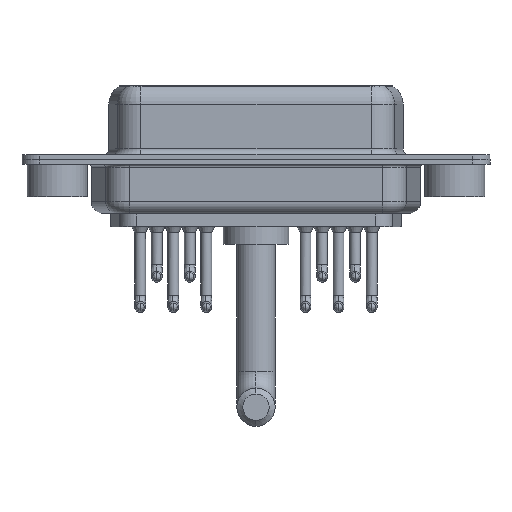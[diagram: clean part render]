
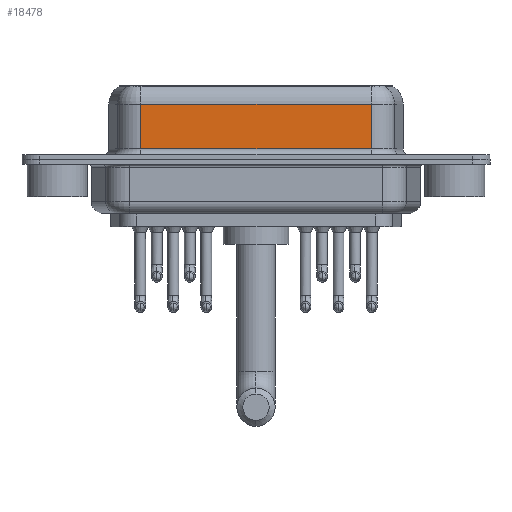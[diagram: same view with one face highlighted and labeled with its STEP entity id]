
A CAD part, front view. The second image highlights one B-rep face of the part: STEP entity #18478.
In plain terms, the highlighted planar face has unit normal (0, -1, 0).
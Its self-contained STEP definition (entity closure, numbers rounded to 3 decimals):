
#212 = VECTOR ( 'NONE', #18120, 1000. ) ;
#762 = CARTESIAN_POINT ( 'NONE',  ( 7.013, -3.95, 4.65 ) ) ;
#2503 = PLANE ( 'NONE',  #17498 ) ;
#2688 = VERTEX_POINT ( 'NONE', #15954 ) ;
#2879 = VERTEX_POINT ( 'NONE', #17060 ) ;
#2999 = EDGE_CURVE ( 'NONE', #7984, #10049, #8104, .T. ) ;
#3759 = ORIENTED_EDGE ( 'NONE', *, *, #16179, .F. ) ;
#4712 = CARTESIAN_POINT ( 'NONE',  ( 7.013, -3.95, 0.9 ) ) ;
#4787 = DIRECTION ( 'NONE',  ( -1., 0., 0. ) ) ;
#5198 = VECTOR ( 'NONE', #11987, 1000. ) ;
#5948 = EDGE_CURVE ( 'NONE', #2879, #7984, #13646, .T. ) ;
#6140 = LINE ( 'NONE', #17648, #5198 ) ;
#6589 = VECTOR ( 'NONE', #16693, 1000. ) ;
#6753 = FACE_OUTER_BOUND ( 'NONE', #17752, .T. ) ;
#7984 = VERTEX_POINT ( 'NONE', #762 ) ;
#8010 = LINE ( 'NONE', #13747, #6589 ) ;
#8104 = LINE ( 'NONE', #13842, #212 ) ;
#8258 = DIRECTION ( 'NONE',  ( 0., 1., 0. ) ) ;
#9667 = CARTESIAN_POINT ( 'NONE',  ( 26.287, -3.95, 6.4 ) ) ;
#10049 = VERTEX_POINT ( 'NONE', #4712 ) ;
#11621 = EDGE_CURVE ( 'NONE', #10049, #2688, #6140, .T. ) ;
#11987 = DIRECTION ( 'NONE',  ( 1., 0., 0. ) ) ;
#13646 = LINE ( 'NONE', #17723, #17110 ) ;
#13747 = CARTESIAN_POINT ( 'NONE',  ( 26.287, -3.95, 6.4 ) ) ;
#13842 = CARTESIAN_POINT ( 'NONE',  ( 7.013, -3.95, 6.4 ) ) ;
#15729 = ORIENTED_EDGE ( 'NONE', *, *, #11621, .T. ) ;
#15954 = CARTESIAN_POINT ( 'NONE',  ( 26.287, -3.95, 0.9 ) ) ;
#16179 = EDGE_CURVE ( 'NONE', #2879, #2688, #8010, .T. ) ;
#16663 = DIRECTION ( 'NONE',  ( 0., 0., 1. ) ) ;
#16693 = DIRECTION ( 'NONE',  ( 0., 0., -1. ) ) ;
#17060 = CARTESIAN_POINT ( 'NONE',  ( 26.287, -3.95, 4.65 ) ) ;
#17110 = VECTOR ( 'NONE', #4787, 1000. ) ;
#17498 = AXIS2_PLACEMENT_3D ( 'NONE', #9667, #8258, #16663 ) ;
#17648 = CARTESIAN_POINT ( 'NONE',  ( 26.287, -3.95, 0.9 ) ) ;
#17723 = CARTESIAN_POINT ( 'NONE',  ( 26.287, -3.95, 4.65 ) ) ;
#17752 = EDGE_LOOP ( 'NONE', ( #3759, #18330, #17755, #15729 ) ) ;
#17755 = ORIENTED_EDGE ( 'NONE', *, *, #2999, .T. ) ;
#18120 = DIRECTION ( 'NONE',  ( 0., 0., -1. ) ) ;
#18330 = ORIENTED_EDGE ( 'NONE', *, *, #5948, .T. ) ;
#18478 = ADVANCED_FACE ( 'NONE', ( #6753 ), #2503, .F. ) ;
